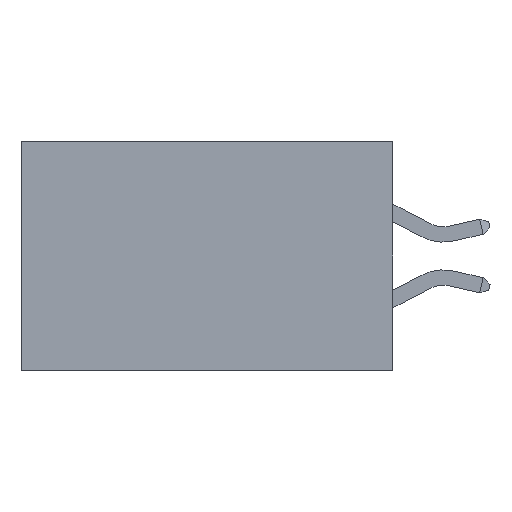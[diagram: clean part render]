
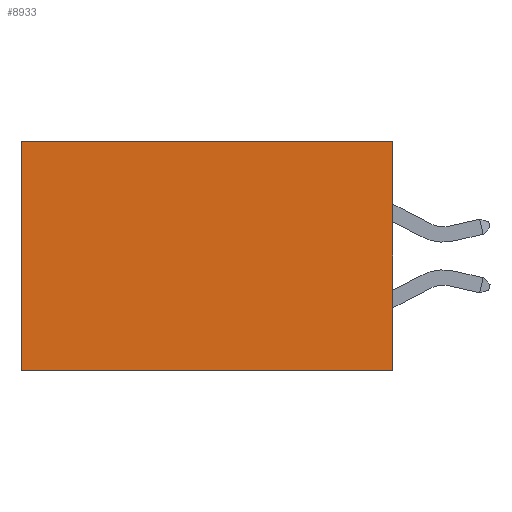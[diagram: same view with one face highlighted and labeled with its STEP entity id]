
A CAD part, left-side view. The second image highlights one B-rep face of the part: STEP entity #8933.
In plain terms, the highlighted planar face has unit normal (-1, 0, 0).
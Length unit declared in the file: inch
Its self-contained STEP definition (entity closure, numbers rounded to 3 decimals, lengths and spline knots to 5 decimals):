
#487 = CARTESIAN_POINT ( 'NONE',  ( 0.2875, 0., 0. ) ) ;
#1064 = EDGE_LOOP ( 'NONE', ( #22122, #4653, #8064, #9183 ) ) ;
#1131 = VECTOR ( 'NONE', #24684, 39.37008 ) ;
#2909 = VECTOR ( 'NONE', #9280, 39.37008 ) ;
#3460 = LINE ( 'NONE', #487, #20917 ) ;
#3524 = EDGE_CURVE ( 'NONE', #8642, #8893, #19242, .T. ) ;
#4295 = LINE ( 'NONE', #22175, #2909 ) ;
#4653 = ORIENTED_EDGE ( 'NONE', *, *, #3524, .F. ) ;
#6437 = CARTESIAN_POINT ( 'NONE',  ( 0.2875, 0., 0. ) ) ;
#7026 = CARTESIAN_POINT ( 'NONE',  ( 0.2875, 0., -0.37 ) ) ;
#7385 = LINE ( 'NONE', #11385, #8980 ) ;
#7501 = DIRECTION ( 'NONE',  ( 1., 0., 0. ) ) ;
#7781 = CARTESIAN_POINT ( 'NONE',  ( 0.2875, 0., 0. ) ) ;
#8064 = ORIENTED_EDGE ( 'NONE', *, *, #19955, .F. ) ;
#8066 = VERTEX_POINT ( 'NONE', #6437 ) ;
#8642 = VERTEX_POINT ( 'NONE', #27543 ) ;
#8893 = VERTEX_POINT ( 'NONE', #27171 ) ;
#8933 = ADVANCED_FACE ( 'NONE', ( #23195 ), #20499, .F. ) ;
#8980 = VECTOR ( 'NONE', #18440, 39.37008 ) ;
#9183 = ORIENTED_EDGE ( 'NONE', *, *, #27201, .T. ) ;
#9280 = DIRECTION ( 'NONE',  ( 0., 0., -1. ) ) ;
#10075 = EDGE_CURVE ( 'NONE', #12301, #8893, #4295, .T. ) ;
#11385 = CARTESIAN_POINT ( 'NONE',  ( 0.2875, 0., 0. ) ) ;
#12301 = VERTEX_POINT ( 'NONE', #14835 ) ;
#14835 = CARTESIAN_POINT ( 'NONE',  ( 0.2875, 0.6, 0. ) ) ;
#15784 = DIRECTION ( 'NONE',  ( 0., 0., -1. ) ) ;
#18440 = DIRECTION ( 'NONE',  ( 0., 1., 0. ) ) ;
#19242 = LINE ( 'NONE', #7026, #1131 ) ;
#19955 = EDGE_CURVE ( 'NONE', #8066, #8642, #3460, .T. ) ;
#20499 = PLANE ( 'NONE',  #24810 ) ;
#20917 = VECTOR ( 'NONE', #15784, 39.37008 ) ;
#22122 = ORIENTED_EDGE ( 'NONE', *, *, #10075, .T. ) ;
#22175 = CARTESIAN_POINT ( 'NONE',  ( 0.2875, 0.6, 0. ) ) ;
#23006 = DIRECTION ( 'NONE',  ( 0., 0., -1. ) ) ;
#23195 = FACE_OUTER_BOUND ( 'NONE', #1064, .T. ) ;
#24684 = DIRECTION ( 'NONE',  ( 0., 1., 0. ) ) ;
#24810 = AXIS2_PLACEMENT_3D ( 'NONE', #7781, #7501, #23006 ) ;
#27171 = CARTESIAN_POINT ( 'NONE',  ( 0.2875, 0.6, -0.37 ) ) ;
#27201 = EDGE_CURVE ( 'NONE', #8066, #12301, #7385, .T. ) ;
#27543 = CARTESIAN_POINT ( 'NONE',  ( 0.2875, 0., -0.37 ) ) ;
